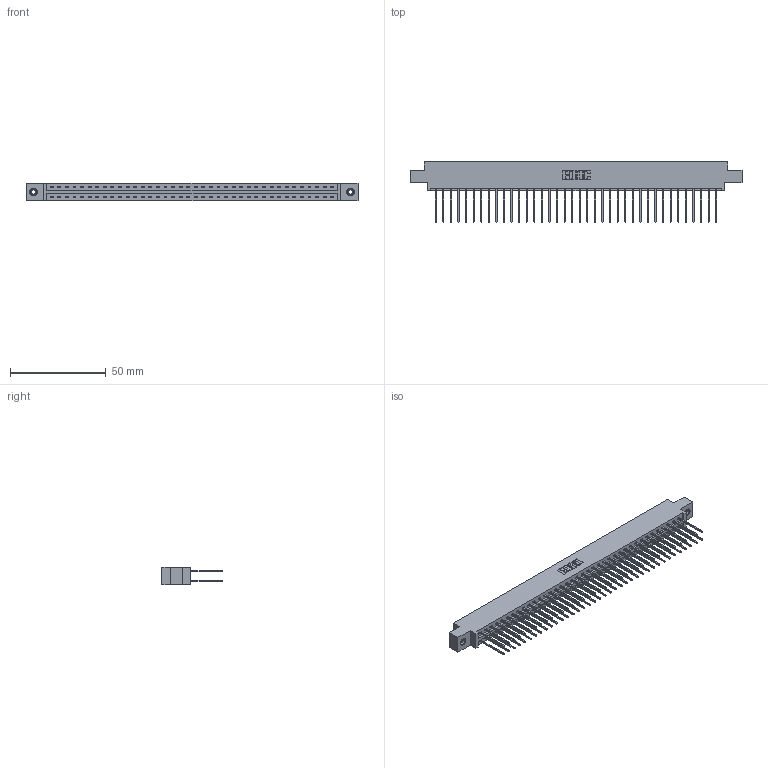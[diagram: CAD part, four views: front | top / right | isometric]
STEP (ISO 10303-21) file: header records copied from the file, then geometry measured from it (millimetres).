
FILE_DESCRIPTION (( 'STEP AP203' ), '1' );
FILE_NAME ('337-076-542-808.STEP', '2019-10-15T13:27:31', ( '' ), ( '' ), 'SwSTEP 2.0', 'SolidWorks 2016', '' );
FILE_SCHEMA (( 'CONFIG_CONTROL_DESIGN' ));
Length unit declared in the file: inch
Products named in the file (4): 345-292-001_345-293-142; 345-250-001_345-250-003-102; 337 Part_0.170 Offset - 0.156 Dia-TI; 337-076-542-808
Assembly tree (79 placements, depth 2):
  337-076-542-808
    337 Part_0.170 Offset - 0.156 Dia-TI
    345-292-001_345-293-142  x76
    345-250-001_345-250-003-102  x2
Bounding box: 173.58 x 31.63 x 9.4 mm (x, y, z)
Volume: 18470.6 mm3; surface area: 22740.2 mm2
Topology: 79 solids, 79 shells, 4282 faces, 12695 edges, 8354 vertices
Faces by surface type: plane 2994, cylinder 1272, cone 12, torus 4
Entity records: 31316 total; most frequent: CARTESIAN_POINT 5261, ORIENTED_EDGE 5190, DIRECTION 4513, EDGE_CURVE 2595, VECTOR 2447, LINE 2447, VERTEX_POINT 1724, AXIS2_PLACEMENT_3D 1033
